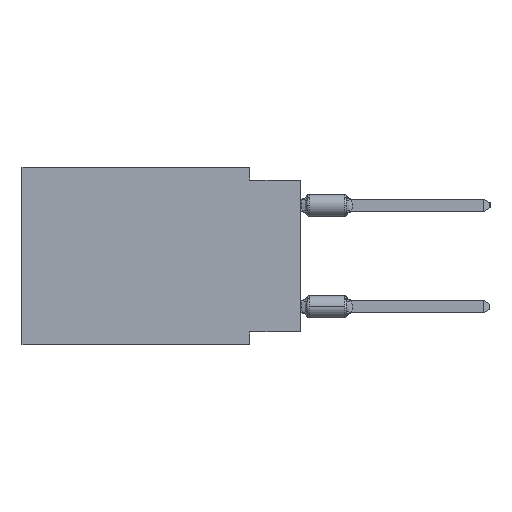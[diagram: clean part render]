
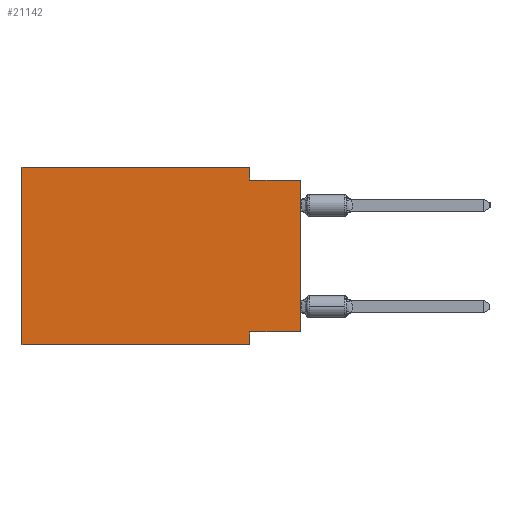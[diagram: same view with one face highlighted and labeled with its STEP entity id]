
A CAD part, left-side view. The second image highlights one B-rep face of the part: STEP entity #21142.
In plain terms, the highlighted planar face has unit normal (-1, 0, 0).
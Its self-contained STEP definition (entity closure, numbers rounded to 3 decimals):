
#178 = CARTESIAN_POINT ( 'NONE',  ( 0., 0., 0. ) ) ;
#258 = PLANE ( 'NONE',  #3622 ) ;
#1209 = EDGE_CURVE ( 'NONE', #8297, #19162, #13843, .T. ) ;
#1224 = LINE ( 'NONE', #9309, #10702 ) ;
#1531 = EDGE_CURVE ( 'NONE', #11137, #4641, #21129, .T. ) ;
#1717 = VECTOR ( 'NONE', #21723, 1000. ) ;
#1885 = VECTOR ( 'NONE', #22512, 1000. ) ;
#2016 = DIRECTION ( 'NONE',  ( 0., 0., 1. ) ) ;
#2084 = VECTOR ( 'NONE', #17395, 1000. ) ;
#2424 = VECTOR ( 'NONE', #26122, 1000. ) ;
#2712 = CARTESIAN_POINT ( 'NONE',  ( 0., 2.54, -8.255 ) ) ;
#2933 = CARTESIAN_POINT ( 'NONE',  ( 0., 2.54, -8.89 ) ) ;
#3622 = AXIS2_PLACEMENT_3D ( 'NONE', #12471, #6484, #10196 ) ;
#3682 = EDGE_CURVE ( 'NONE', #24795, #23725, #22232, .T. ) ;
#4641 = VERTEX_POINT ( 'NONE', #18938 ) ;
#5506 = CARTESIAN_POINT ( 'NONE',  ( 0., 13.97, 0. ) ) ;
#5890 = ORIENTED_EDGE ( 'NONE', *, *, #23933, .F. ) ;
#5940 = CARTESIAN_POINT ( 'NONE',  ( 0., 2.54, 0. ) ) ;
#6064 = EDGE_CURVE ( 'NONE', #17838, #10098, #17899, .T. ) ;
#6484 = DIRECTION ( 'NONE',  ( 1., 0., 0. ) ) ;
#6788 = CARTESIAN_POINT ( 'NONE',  ( 0., 2.54, 0. ) ) ;
#8297 = VERTEX_POINT ( 'NONE', #11659 ) ;
#9309 = CARTESIAN_POINT ( 'NONE',  ( 0., 0., -0.635 ) ) ;
#10098 = VERTEX_POINT ( 'NONE', #14147 ) ;
#10142 = EDGE_LOOP ( 'NONE', ( #17149, #5890, #14775, #10784, #25448, #22473, #15119, #25736 ) ) ;
#10196 = DIRECTION ( 'NONE',  ( 0., 0., -1. ) ) ;
#10702 = VECTOR ( 'NONE', #23643, 1000. ) ;
#10784 = ORIENTED_EDGE ( 'NONE', *, *, #14678, .F. ) ;
#11137 = VERTEX_POINT ( 'NONE', #2712 ) ;
#11659 = CARTESIAN_POINT ( 'NONE',  ( 0., 0., -8.255 ) ) ;
#12471 = CARTESIAN_POINT ( 'NONE',  ( 0., 13.97, 0. ) ) ;
#12861 = FACE_OUTER_BOUND ( 'NONE', #10142, .T. ) ;
#13843 = LINE ( 'NONE', #178, #22858 ) ;
#14147 = CARTESIAN_POINT ( 'NONE',  ( 0., 2.54, -0.635 ) ) ;
#14411 = CARTESIAN_POINT ( 'NONE',  ( 0., 0., -8.255 ) ) ;
#14678 = EDGE_CURVE ( 'NONE', #23725, #17838, #25818, .T. ) ;
#14739 = EDGE_CURVE ( 'NONE', #24795, #4641, #21977, .T. ) ;
#14775 = ORIENTED_EDGE ( 'NONE', *, *, #6064, .F. ) ;
#15119 = ORIENTED_EDGE ( 'NONE', *, *, #1531, .F. ) ;
#15551 = CARTESIAN_POINT ( 'NONE',  ( 0., 0., -0.635 ) ) ;
#16146 = VECTOR ( 'NONE', #26084, 1000. ) ;
#17149 = ORIENTED_EDGE ( 'NONE', *, *, #1209, .T. ) ;
#17395 = DIRECTION ( 'NONE',  ( 0., 0., -1. ) ) ;
#17427 = VECTOR ( 'NONE', #26203, 1000. ) ;
#17838 = VERTEX_POINT ( 'NONE', #6788 ) ;
#17899 = LINE ( 'NONE', #5940, #2424 ) ;
#17993 = CARTESIAN_POINT ( 'NONE',  ( 0., 13.97, -8.89 ) ) ;
#18938 = CARTESIAN_POINT ( 'NONE',  ( 0., 2.54, -8.89 ) ) ;
#18958 = CARTESIAN_POINT ( 'NONE',  ( 0., 13.97, -8.89 ) ) ;
#19162 = VERTEX_POINT ( 'NONE', #15551 ) ;
#20324 = EDGE_CURVE ( 'NONE', #8297, #11137, #24495, .T. ) ;
#21129 = LINE ( 'NONE', #2933, #2084 ) ;
#21142 = ADVANCED_FACE ( 'NONE', ( #12861 ), #258, .F. ) ;
#21723 = DIRECTION ( 'NONE',  ( 0., -1., 0. ) ) ;
#21977 = LINE ( 'NONE', #17993, #16146 ) ;
#22104 = CARTESIAN_POINT ( 'NONE',  ( 0., 13.97, 0. ) ) ;
#22232 = LINE ( 'NONE', #22104, #17427 ) ;
#22473 = ORIENTED_EDGE ( 'NONE', *, *, #14739, .T. ) ;
#22512 = DIRECTION ( 'NONE',  ( 0., 1., 0. ) ) ;
#22858 = VECTOR ( 'NONE', #2016, 1000. ) ;
#23643 = DIRECTION ( 'NONE',  ( 0., -1., 0. ) ) ;
#23725 = VERTEX_POINT ( 'NONE', #25836 ) ;
#23933 = EDGE_CURVE ( 'NONE', #10098, #19162, #1224, .T. ) ;
#24495 = LINE ( 'NONE', #14411, #1885 ) ;
#24795 = VERTEX_POINT ( 'NONE', #18958 ) ;
#25448 = ORIENTED_EDGE ( 'NONE', *, *, #3682, .F. ) ;
#25736 = ORIENTED_EDGE ( 'NONE', *, *, #20324, .F. ) ;
#25818 = LINE ( 'NONE', #5506, #1717 ) ;
#25836 = CARTESIAN_POINT ( 'NONE',  ( 0., 13.97, 0. ) ) ;
#26084 = DIRECTION ( 'NONE',  ( 0., -1., 0. ) ) ;
#26122 = DIRECTION ( 'NONE',  ( 0., 0., -1. ) ) ;
#26203 = DIRECTION ( 'NONE',  ( 0., 0., 1. ) ) ;
